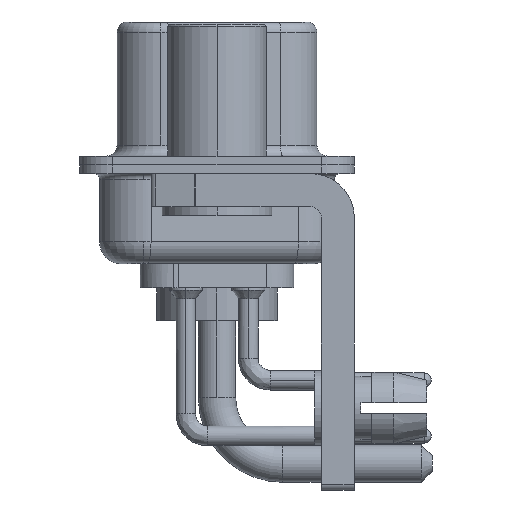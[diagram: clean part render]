
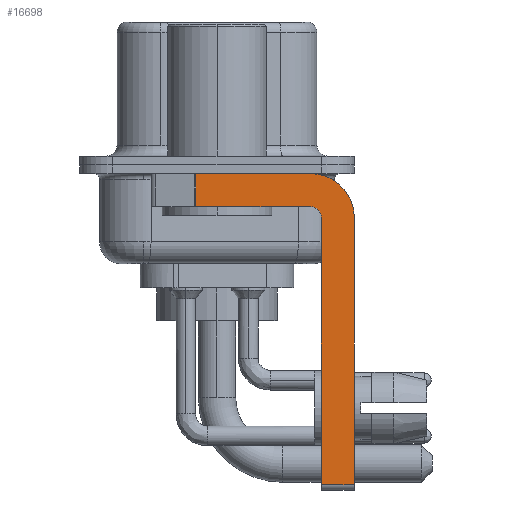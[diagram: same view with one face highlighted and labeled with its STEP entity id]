
A CAD part, left-side view. The second image highlights one B-rep face of the part: STEP entity #16698.
In plain terms, the highlighted planar face has unit normal (-1, 0, 0).
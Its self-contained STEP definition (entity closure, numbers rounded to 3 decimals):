
#190 = CARTESIAN_POINT ( 'NONE',  ( -2.9, -6.25, -2.4 ) ) ;
#678 = VERTEX_POINT ( 'NONE', #190 ) ;
#1348 = CARTESIAN_POINT ( 'NONE',  ( -2.9, -4.25, -2.4 ) ) ;
#1519 = DIRECTION ( 'NONE',  ( 1., 0., 0. ) ) ;
#1911 = CARTESIAN_POINT ( 'NONE',  ( -2.9, 0.978, -1.9 ) ) ;
#2128 = CARTESIAN_POINT ( 'NONE',  ( -2.9, -4.25, -1.9 ) ) ;
#2165 = CARTESIAN_POINT ( 'NONE',  ( -2.9, -4.25, -2.4 ) ) ;
#2208 = CIRCLE ( 'NONE', #6802, 0.5 ) ;
#2383 = CARTESIAN_POINT ( 'NONE',  ( -2.9, -4.25, -1.9 ) ) ;
#2898 = DIRECTION ( 'NONE',  ( 0., 0., -1. ) ) ;
#3101 = LINE ( 'NONE', #14023, #12371 ) ;
#3263 = EDGE_CURVE ( 'NONE', #678, #15071, #3101, .T. ) ;
#3771 = ORIENTED_EDGE ( 'NONE', *, *, #10167, .F. ) ;
#4316 = ORIENTED_EDGE ( 'NONE', *, *, #14052, .F. ) ;
#5043 = FACE_OUTER_BOUND ( 'NONE', #17560, .T. ) ;
#5060 = EDGE_CURVE ( 'NONE', #17723, #10846, #2208, .T. ) ;
#5118 = CARTESIAN_POINT ( 'NONE',  ( -2.9, 3., -0.4 ) ) ;
#5186 = EDGE_CURVE ( 'NONE', #15845, #15071, #11437, .T. ) ;
#6802 = AXIS2_PLACEMENT_3D ( 'NONE', #2165, #16668, #9200 ) ;
#7704 = DIRECTION ( 'NONE',  ( 0., 0., 1. ) ) ;
#7721 = EDGE_CURVE ( 'NONE', #10846, #9724, #14716, .T. ) ;
#8129 = DIRECTION ( 'NONE',  ( 1., 0., 0. ) ) ;
#8299 = VECTOR ( 'NONE', #12979, 1000. ) ;
#9200 = DIRECTION ( 'NONE',  ( 0., 0., 1. ) ) ;
#9207 = ORIENTED_EDGE ( 'NONE', *, *, #3263, .F. ) ;
#9367 = CARTESIAN_POINT ( 'NONE',  ( -2.9, -4.75, -14.55 ) ) ;
#9724 = VERTEX_POINT ( 'NONE', #16284 ) ;
#9922 = CARTESIAN_POINT ( 'NONE',  ( -2.9, -4.75, -2.4 ) ) ;
#10167 = EDGE_CURVE ( 'NONE', #13389, #678, #14086, .T. ) ;
#10277 = CARTESIAN_POINT ( 'NONE',  ( -2.9, -6.25, -14.55 ) ) ;
#10846 = VERTEX_POINT ( 'NONE', #2383 ) ;
#11190 = CARTESIAN_POINT ( 'NONE',  ( -2.9, -4.25, -0.4 ) ) ;
#11437 = LINE ( 'NONE', #14752, #8299 ) ;
#11678 = VECTOR ( 'NONE', #20411, 1000. ) ;
#11753 = CARTESIAN_POINT ( 'NONE',  ( -2.9, -4.75, -14.8 ) ) ;
#12183 = ORIENTED_EDGE ( 'NONE', *, *, #5186, .T. ) ;
#12303 = EDGE_CURVE ( 'NONE', #17060, #13389, #21150, .T. ) ;
#12371 = VECTOR ( 'NONE', #17364, 1000. ) ;
#12639 = VECTOR ( 'NONE', #22817, 1000. ) ;
#12979 = DIRECTION ( 'NONE',  ( 0., -1., 0. ) ) ;
#13275 = ORIENTED_EDGE ( 'NONE', *, *, #12303, .F. ) ;
#13389 = VERTEX_POINT ( 'NONE', #11190 ) ;
#13398 = VECTOR ( 'NONE', #7704, 1000. ) ;
#14023 = CARTESIAN_POINT ( 'NONE',  ( -2.9, -6.25, -2.4 ) ) ;
#14052 = EDGE_CURVE ( 'NONE', #15845, #17723, #18758, .T. ) ;
#14086 = CIRCLE ( 'NONE', #17114, 2. ) ;
#14716 = LINE ( 'NONE', #2128, #11678 ) ;
#14752 = CARTESIAN_POINT ( 'NONE',  ( -2.9, -4.25, -14.55 ) ) ;
#15071 = VERTEX_POINT ( 'NONE', #10277 ) ;
#15845 = VERTEX_POINT ( 'NONE', #9367 ) ;
#16129 = DIRECTION ( 'NONE',  ( 0., 0., -1. ) ) ;
#16284 = CARTESIAN_POINT ( 'NONE',  ( -2.9, 0.978, -1.9 ) ) ;
#16668 = DIRECTION ( 'NONE',  ( -1., 0., 0. ) ) ;
#16698 = ADVANCED_FACE ( 'NONE', ( #5043 ), #17636, .F. ) ;
#16751 = DIRECTION ( 'NONE',  ( 0., 0., -1. ) ) ;
#17060 = VERTEX_POINT ( 'NONE', #19036 ) ;
#17114 = AXIS2_PLACEMENT_3D ( 'NONE', #23371, #1519, #16129 ) ;
#17364 = DIRECTION ( 'NONE',  ( 0., 0., -1. ) ) ;
#17560 = EDGE_LOOP ( 'NONE', ( #13275, #20782, #21972, #22809, #4316, #12183, #9207, #3771 ) ) ;
#17636 = PLANE ( 'NONE',  #19192 ) ;
#17723 = VERTEX_POINT ( 'NONE', #9922 ) ;
#18758 = LINE ( 'NONE', #11753, #13398 ) ;
#19036 = CARTESIAN_POINT ( 'NONE',  ( -2.9, 0.978, -0.4 ) ) ;
#19192 = AXIS2_PLACEMENT_3D ( 'NONE', #1348, #8129, #2898 ) ;
#20073 = LINE ( 'NONE', #1911, #21959 ) ;
#20411 = DIRECTION ( 'NONE',  ( 0., 1., 0. ) ) ;
#20782 = ORIENTED_EDGE ( 'NONE', *, *, #21956, .T. ) ;
#21150 = LINE ( 'NONE', #5118, #12639 ) ;
#21956 = EDGE_CURVE ( 'NONE', #17060, #9724, #20073, .T. ) ;
#21959 = VECTOR ( 'NONE', #16751, 1000. ) ;
#21972 = ORIENTED_EDGE ( 'NONE', *, *, #7721, .F. ) ;
#22809 = ORIENTED_EDGE ( 'NONE', *, *, #5060, .F. ) ;
#22817 = DIRECTION ( 'NONE',  ( 0., -1., 0. ) ) ;
#23371 = CARTESIAN_POINT ( 'NONE',  ( -2.9, -4.25, -2.4 ) ) ;
